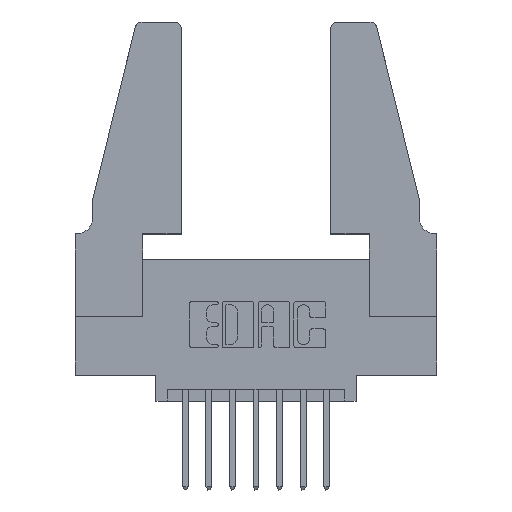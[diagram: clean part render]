
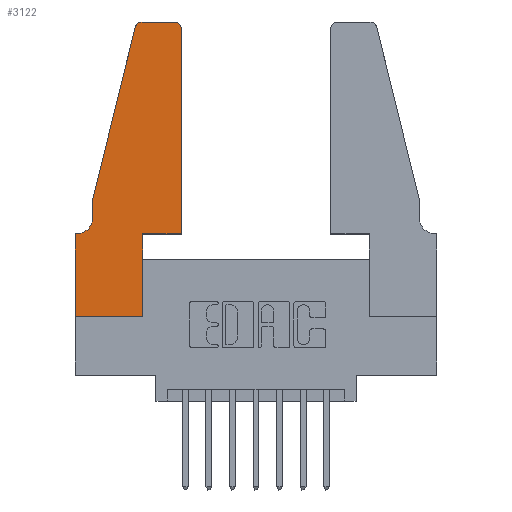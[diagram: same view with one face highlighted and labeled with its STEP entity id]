
A CAD part, top view. The second image highlights one B-rep face of the part: STEP entity #3122.
In plain terms, the highlighted planar face has unit normal (0, 0, 1).
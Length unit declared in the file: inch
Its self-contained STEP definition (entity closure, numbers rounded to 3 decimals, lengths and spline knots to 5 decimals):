
#9 = CARTESIAN_POINT ( 'NONE',  ( 0., 0., 0.37 ) ) ;
#387 = VERTEX_POINT ( 'NONE', #9679 ) ;
#1081 = EDGE_CURVE ( 'NONE', #10692, #9118, #6007, .T. ) ;
#1255 = VECTOR ( 'NONE', #8729, 39.37008 ) ;
#1286 = CARTESIAN_POINT ( 'NONE',  ( 0.2865, 0.35, 0.37 ) ) ;
#1419 = LINE ( 'NONE', #6386, #2474 ) ;
#1549 = VECTOR ( 'NONE', #12523, 39.37008 ) ;
#1592 = ORIENTED_EDGE ( 'NONE', *, *, #9480, .T. ) ;
#1736 = VECTOR ( 'NONE', #6994, 39.37008 ) ;
#1788 = CARTESIAN_POINT ( 'NONE',  ( 0.4505, 0.35, 0.37 ) ) ;
#1895 = CARTESIAN_POINT ( 'NONE',  ( 0.0755, 0.5, 0.37 ) ) ;
#2431 = ORIENTED_EDGE ( 'NONE', *, *, #4867, .T. ) ;
#2474 = VECTOR ( 'NONE', #8384, 39.37008 ) ;
#2505 = AXIS2_PLACEMENT_3D ( 'NONE', #4413, #2609, #11324 ) ;
#2609 = DIRECTION ( 'NONE',  ( 0., 0., -1. ) ) ;
#2857 = VERTEX_POINT ( 'NONE', #10672 ) ;
#3044 = VERTEX_POINT ( 'NONE', #6265 ) ;
#3122 = ADVANCED_FACE ( 'NONE', ( #5950 ), #6985, .T. ) ;
#3198 = DIRECTION ( 'NONE',  ( 1., 0., 0. ) ) ;
#3211 = DIRECTION ( 'NONE',  ( -0.239, -0.971, 0. ) ) ;
#3546 = CARTESIAN_POINT ( 'NONE',  ( 0.0755, 0.5, 0.37 ) ) ;
#3687 = VECTOR ( 'NONE', #9660, 39.37008 ) ;
#4026 = EDGE_CURVE ( 'NONE', #10021, #4143, #10669, .T. ) ;
#4066 = CARTESIAN_POINT ( 'NONE',  ( 0.0755, 0.42, 0.37 ) ) ;
#4143 = VERTEX_POINT ( 'NONE', #9851 ) ;
#4256 = CARTESIAN_POINT ( 'NONE',  ( 0.0755, 0.35, 0.37 ) ) ;
#4260 = LINE ( 'NONE', #9, #1255 ) ;
#4277 = CARTESIAN_POINT ( 'NONE',  ( 0., 0.35, 0.37 ) ) ;
#4413 = CARTESIAN_POINT ( 'NONE',  ( 0.0055, 0.42, 0.37 ) ) ;
#4490 = AXIS2_PLACEMENT_3D ( 'NONE', #4277, #10171, #6123 ) ;
#4493 = ORIENTED_EDGE ( 'NONE', *, *, #7020, .T. ) ;
#4652 = EDGE_CURVE ( 'NONE', #9118, #5352, #8554, .T. ) ;
#4716 = CARTESIAN_POINT ( 'NONE',  ( 0.4505, 0.35, 0.37 ) ) ;
#4867 = EDGE_CURVE ( 'NONE', #10558, #9511, #10518, .T. ) ;
#4884 = EDGE_CURVE ( 'NONE', #387, #2857, #10086, .T. ) ;
#5171 = CARTESIAN_POINT ( 'NONE',  ( 0.25487, 1.22718, 0.37 ) ) ;
#5318 = CARTESIAN_POINT ( 'NONE',  ( 0.4505, 1.22, 0.37 ) ) ;
#5352 = VERTEX_POINT ( 'NONE', #5318 ) ;
#5464 = EDGE_CURVE ( 'NONE', #4143, #7041, #4260, .T. ) ;
#5482 = ORIENTED_EDGE ( 'NONE', *, *, #4884, .T. ) ;
#5638 = DIRECTION ( 'NONE',  ( 1., 0., 0. ) ) ;
#5906 = EDGE_CURVE ( 'NONE', #3044, #10692, #8521, .T. ) ;
#5912 = DIRECTION ( 'NONE',  ( 0., 0., 1. ) ) ;
#5950 = FACE_OUTER_BOUND ( 'NONE', #7497, .T. ) ;
#6007 = LINE ( 'NONE', #1788, #11645 ) ;
#6123 = DIRECTION ( 'NONE',  ( 1., 0., 0. ) ) ;
#6265 = CARTESIAN_POINT ( 'NONE',  ( 0.2865, 0., 0.37 ) ) ;
#6386 = CARTESIAN_POINT ( 'NONE',  ( 0., 0., 0.37 ) ) ;
#6607 = DIRECTION ( 'NONE',  ( 0., 1., 0. ) ) ;
#6729 = CARTESIAN_POINT ( 'NONE',  ( 0.0055, 0.35, 0.37 ) ) ;
#6908 = EDGE_CURVE ( 'NONE', #5352, #387, #9356, .T. ) ;
#6953 = EDGE_CURVE ( 'NONE', #9511, #10021, #11437, .T. ) ;
#6975 = AXIS2_PLACEMENT_3D ( 'NONE', #8941, #7100, #3198 ) ;
#6985 = PLANE ( 'NONE',  #4490 ) ;
#6994 = DIRECTION ( 'NONE',  ( -1., 0., 0. ) ) ;
#7020 = EDGE_CURVE ( 'NONE', #2857, #10944, #12046, .T. ) ;
#7041 = VERTEX_POINT ( 'NONE', #9759 ) ;
#7100 = DIRECTION ( 'NONE',  ( 0., 0., 1. ) ) ;
#7148 = DIRECTION ( 'NONE',  ( -1., 0., 0. ) ) ;
#7497 = EDGE_LOOP ( 'NONE', ( #5482, #4493, #1592, #2431, #12012, #11667, #9199, #10656, #10980, #10854, #10599, #12374 ) ) ;
#7753 = CARTESIAN_POINT ( 'NONE',  ( 0.2865, 0.35, 0.37 ) ) ;
#8348 = AXIS2_PLACEMENT_3D ( 'NONE', #8832, #5912, #9937 ) ;
#8384 = DIRECTION ( 'NONE',  ( 1., 0., 0. ) ) ;
#8521 = LINE ( 'NONE', #7753, #1549 ) ;
#8554 = LINE ( 'NONE', #4716, #9348 ) ;
#8729 = DIRECTION ( 'NONE',  ( 0., -1., 0. ) ) ;
#8832 = CARTESIAN_POINT ( 'NONE',  ( 0.284, 1.22, 0.37 ) ) ;
#8880 = EDGE_CURVE ( 'NONE', #7041, #3044, #1419, .T. ) ;
#8941 = CARTESIAN_POINT ( 'NONE',  ( 0.4205, 1.22, 0.37 ) ) ;
#9118 = VERTEX_POINT ( 'NONE', #10206 ) ;
#9199 = ORIENTED_EDGE ( 'NONE', *, *, #5464, .T. ) ;
#9348 = VECTOR ( 'NONE', #6607, 39.37008 ) ;
#9356 = CIRCLE ( 'NONE', #6975, 0.03 ) ;
#9480 = EDGE_CURVE ( 'NONE', #10944, #10558, #11234, .T. ) ;
#9494 = VECTOR ( 'NONE', #7148, 39.37008 ) ;
#9511 = VERTEX_POINT ( 'NONE', #4066 ) ;
#9660 = DIRECTION ( 'NONE',  ( 0., -1., 0. ) ) ;
#9679 = CARTESIAN_POINT ( 'NONE',  ( 0.4205, 1.25, 0.37 ) ) ;
#9759 = CARTESIAN_POINT ( 'NONE',  ( 0., 0., 0.37 ) ) ;
#9851 = CARTESIAN_POINT ( 'NONE',  ( 0., 0.35, 0.37 ) ) ;
#9937 = DIRECTION ( 'NONE',  ( 1., 0., 0. ) ) ;
#9943 = CARTESIAN_POINT ( 'NONE',  ( 0.2605, 1.25, 0.37 ) ) ;
#10021 = VERTEX_POINT ( 'NONE', #6729 ) ;
#10086 = LINE ( 'NONE', #9943, #1736 ) ;
#10171 = DIRECTION ( 'NONE',  ( 0., 0., 1. ) ) ;
#10206 = CARTESIAN_POINT ( 'NONE',  ( 0.4505, 0.35, 0.37 ) ) ;
#10518 = LINE ( 'NONE', #1895, #3687 ) ;
#10558 = VERTEX_POINT ( 'NONE', #3546 ) ;
#10599 = ORIENTED_EDGE ( 'NONE', *, *, #4652, .T. ) ;
#10656 = ORIENTED_EDGE ( 'NONE', *, *, #8880, .T. ) ;
#10669 = LINE ( 'NONE', #4256, #9494 ) ;
#10672 = CARTESIAN_POINT ( 'NONE',  ( 0.284, 1.25, 0.37 ) ) ;
#10692 = VERTEX_POINT ( 'NONE', #1286 ) ;
#10854 = ORIENTED_EDGE ( 'NONE', *, *, #1081, .T. ) ;
#10944 = VERTEX_POINT ( 'NONE', #5171 ) ;
#10980 = ORIENTED_EDGE ( 'NONE', *, *, #5906, .T. ) ;
#11004 = CARTESIAN_POINT ( 'NONE',  ( 0.0755, 0.5, 0.37 ) ) ;
#11234 = LINE ( 'NONE', #11004, #12162 ) ;
#11324 = DIRECTION ( 'NONE',  ( -1., 0., 0. ) ) ;
#11437 = CIRCLE ( 'NONE', #2505, 0.07 ) ;
#11645 = VECTOR ( 'NONE', #5638, 39.37008 ) ;
#11667 = ORIENTED_EDGE ( 'NONE', *, *, #4026, .T. ) ;
#12012 = ORIENTED_EDGE ( 'NONE', *, *, #6953, .T. ) ;
#12046 = CIRCLE ( 'NONE', #8348, 0.03 ) ;
#12162 = VECTOR ( 'NONE', #3211, 39.37008 ) ;
#12374 = ORIENTED_EDGE ( 'NONE', *, *, #6908, .T. ) ;
#12523 = DIRECTION ( 'NONE',  ( 0., 1., 0. ) ) ;
